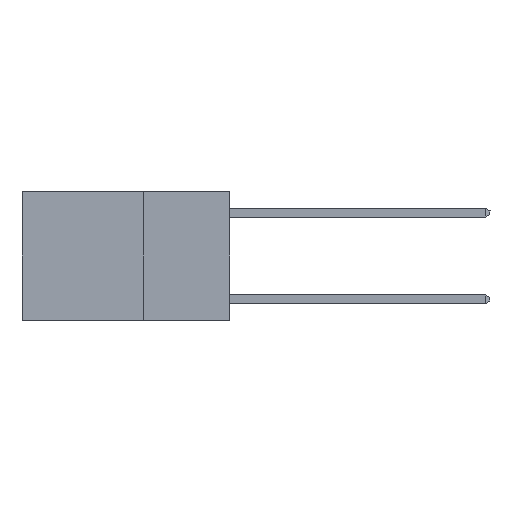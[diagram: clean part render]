
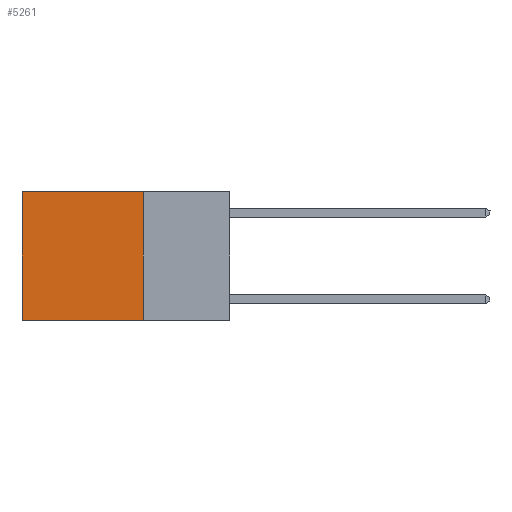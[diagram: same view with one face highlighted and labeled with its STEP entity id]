
A CAD part, left-side view. The second image highlights one B-rep face of the part: STEP entity #5261.
In plain terms, the highlighted planar face has unit normal (-1, 0, 0).
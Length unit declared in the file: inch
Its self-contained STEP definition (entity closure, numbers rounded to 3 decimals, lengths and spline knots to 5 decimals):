
#1081 = DIRECTION ( 'NONE',  ( 0., 0., -1. ) ) ;
#1654 = ORIENTED_EDGE ( 'NONE', *, *, #15342, .T. ) ;
#1673 = ORIENTED_EDGE ( 'NONE', *, *, #8113, .F. ) ;
#1692 = CARTESIAN_POINT ( 'NONE',  ( 0.2625, 0.25, 0. ) ) ;
#1709 = ORIENTED_EDGE ( 'NONE', *, *, #14224, .F. ) ;
#1720 = ORIENTED_EDGE ( 'NONE', *, *, #12920, .T. ) ;
#2349 = CARTESIAN_POINT ( 'NONE',  ( 0.2625, 0.25, -0.37 ) ) ;
#2368 = CARTESIAN_POINT ( 'NONE',  ( 0.2625, 0.25, 0. ) ) ;
#2453 = LINE ( 'NONE', #2983, #3685 ) ;
#2455 = FACE_OUTER_BOUND ( 'NONE', #10218, .T. ) ;
#2983 = CARTESIAN_POINT ( 'NONE',  ( 0.2625, 0.25, 0. ) ) ;
#3685 = VECTOR ( 'NONE', #12041, 39.37008 ) ;
#4213 = VECTOR ( 'NONE', #7593, 39.37008 ) ;
#4232 = LINE ( 'NONE', #12843, #10372 ) ;
#4295 = VERTEX_POINT ( 'NONE', #15910 ) ;
#5261 = ADVANCED_FACE ( 'NONE', ( #2455 ), #13933, .F. ) ;
#5964 = VERTEX_POINT ( 'NONE', #2349 ) ;
#6328 = CARTESIAN_POINT ( 'NONE',  ( 0.2625, 0.25, -0.37 ) ) ;
#6486 = DIRECTION ( 'NONE',  ( 0., 0., -1. ) ) ;
#7593 = DIRECTION ( 'NONE',  ( 0., 1., 0. ) ) ;
#8113 = EDGE_CURVE ( 'NONE', #5964, #4295, #14389, .T. ) ;
#8957 = DIRECTION ( 'NONE',  ( 1., 0., 0. ) ) ;
#10201 = VECTOR ( 'NONE', #15730, 39.37008 ) ;
#10218 = EDGE_LOOP ( 'NONE', ( #1654, #1673, #1709, #1720 ) ) ;
#10372 = VECTOR ( 'NONE', #6486, 39.37008 ) ;
#10816 = CARTESIAN_POINT ( 'NONE',  ( 0.2625, 0.25, 0. ) ) ;
#12041 = DIRECTION ( 'NONE',  ( 0., 1., 0. ) ) ;
#12687 = CARTESIAN_POINT ( 'NONE',  ( 0.2625, 0.6, 0. ) ) ;
#12786 = AXIS2_PLACEMENT_3D ( 'NONE', #2368, #8957, #1081 ) ;
#12843 = CARTESIAN_POINT ( 'NONE',  ( 0.2625, 0.6, 0. ) ) ;
#12920 = EDGE_CURVE ( 'NONE', #12924, #15621, #2453, .T. ) ;
#12924 = VERTEX_POINT ( 'NONE', #10816 ) ;
#13475 = LINE ( 'NONE', #1692, #10201 ) ;
#13933 = PLANE ( 'NONE',  #12786 ) ;
#14224 = EDGE_CURVE ( 'NONE', #12924, #5964, #13475, .T. ) ;
#14389 = LINE ( 'NONE', #6328, #4213 ) ;
#15342 = EDGE_CURVE ( 'NONE', #15621, #4295, #4232, .T. ) ;
#15621 = VERTEX_POINT ( 'NONE', #12687 ) ;
#15730 = DIRECTION ( 'NONE',  ( 0., 0., -1. ) ) ;
#15910 = CARTESIAN_POINT ( 'NONE',  ( 0.2625, 0.6, -0.37 ) ) ;
